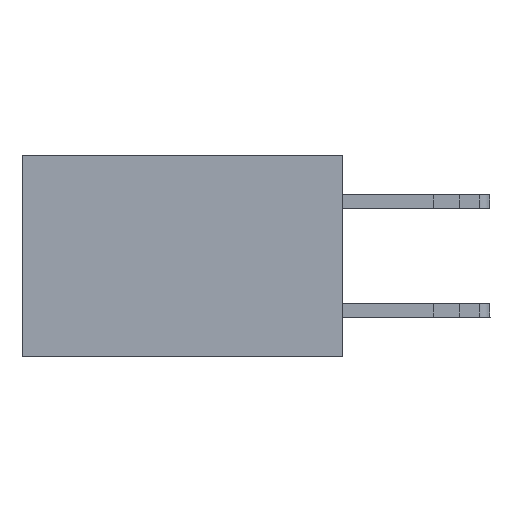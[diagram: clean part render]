
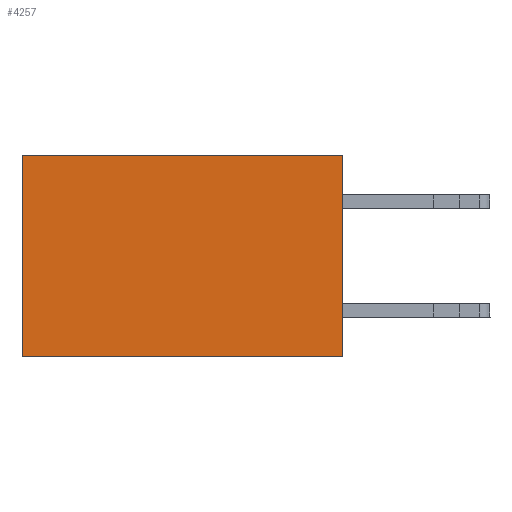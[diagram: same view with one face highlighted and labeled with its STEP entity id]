
A CAD part, left-side view. The second image highlights one B-rep face of the part: STEP entity #4257.
In plain terms, the highlighted planar face has unit normal (-1, 0, 0).
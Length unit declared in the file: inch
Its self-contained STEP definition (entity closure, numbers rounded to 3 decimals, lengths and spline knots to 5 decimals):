
#1540 = VERTEX_POINT ( 'NONE', #13417 ) ;
#1560 = FACE_OUTER_BOUND ( 'NONE', #2710, .T. ) ;
#1605 = VECTOR ( 'NONE', #22966, 39.37008 ) ;
#1868 = DIRECTION ( 'NONE',  ( 1., 0., 0. ) ) ;
#2574 = CARTESIAN_POINT ( 'NONE',  ( 0.277, 0., -0.37 ) ) ;
#2710 = EDGE_LOOP ( 'NONE', ( #15064, #9628, #11223, #23643 ) ) ;
#2724 = CARTESIAN_POINT ( 'NONE',  ( 0.277, 0.59, 0. ) ) ;
#2940 = PLANE ( 'NONE',  #19716 ) ;
#3694 = DIRECTION ( 'NONE',  ( 0., 1., 0. ) ) ;
#4257 = ADVANCED_FACE ( 'NONE', ( #1560 ), #2940, .F. ) ;
#4266 = LINE ( 'NONE', #24067, #14163 ) ;
#4541 = CARTESIAN_POINT ( 'NONE',  ( 0.277, 0.59, -0.37 ) ) ;
#6861 = EDGE_CURVE ( 'NONE', #23003, #1540, #20636, .T. ) ;
#7071 = LINE ( 'NONE', #24733, #1605 ) ;
#7562 = EDGE_CURVE ( 'NONE', #10023, #23003, #4266, .T. ) ;
#8469 = DIRECTION ( 'NONE',  ( 0., 0., -1. ) ) ;
#9628 = ORIENTED_EDGE ( 'NONE', *, *, #18269, .F. ) ;
#10013 = DIRECTION ( 'NONE',  ( 0., 0., -1. ) ) ;
#10023 = VERTEX_POINT ( 'NONE', #10405 ) ;
#10300 = VECTOR ( 'NONE', #10013, 39.37008 ) ;
#10405 = CARTESIAN_POINT ( 'NONE',  ( 0.277, 0., 0. ) ) ;
#11223 = ORIENTED_EDGE ( 'NONE', *, *, #25273, .F. ) ;
#11253 = CARTESIAN_POINT ( 'NONE',  ( 0.277, 0., -0.37 ) ) ;
#12965 = LINE ( 'NONE', #15521, #23236 ) ;
#13417 = CARTESIAN_POINT ( 'NONE',  ( 0.277, 0.59, -0.37 ) ) ;
#13619 = VERTEX_POINT ( 'NONE', #11253 ) ;
#14163 = VECTOR ( 'NONE', #24765, 39.37008 ) ;
#15064 = ORIENTED_EDGE ( 'NONE', *, *, #6861, .T. ) ;
#15521 = CARTESIAN_POINT ( 'NONE',  ( 0.277, 0., -0.37 ) ) ;
#18269 = EDGE_CURVE ( 'NONE', #13619, #1540, #12965, .T. ) ;
#19716 = AXIS2_PLACEMENT_3D ( 'NONE', #2574, #1868, #8469 ) ;
#20636 = LINE ( 'NONE', #4541, #10300 ) ;
#22966 = DIRECTION ( 'NONE',  ( 0., 0., -1. ) ) ;
#23003 = VERTEX_POINT ( 'NONE', #2724 ) ;
#23236 = VECTOR ( 'NONE', #3694, 39.37008 ) ;
#23643 = ORIENTED_EDGE ( 'NONE', *, *, #7562, .T. ) ;
#24067 = CARTESIAN_POINT ( 'NONE',  ( 0.277, 0., 0. ) ) ;
#24733 = CARTESIAN_POINT ( 'NONE',  ( 0.277, 0., -0.37 ) ) ;
#24765 = DIRECTION ( 'NONE',  ( 0., 1., 0. ) ) ;
#25273 = EDGE_CURVE ( 'NONE', #10023, #13619, #7071, .T. ) ;
